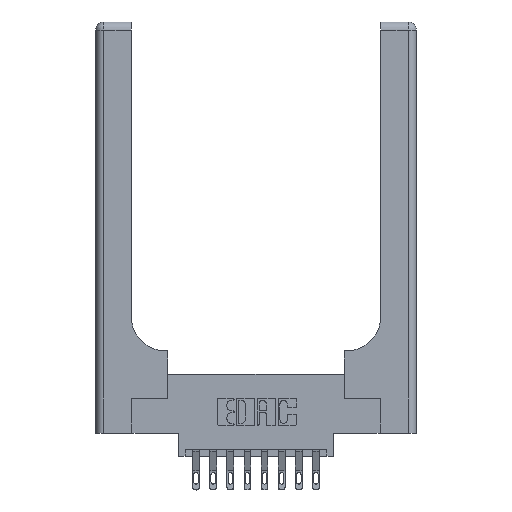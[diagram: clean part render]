
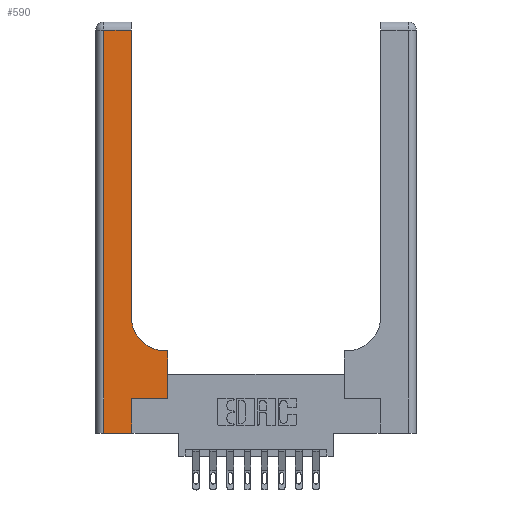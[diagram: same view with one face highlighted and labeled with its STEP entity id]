
A CAD part, top view. The second image highlights one B-rep face of the part: STEP entity #590.
In plain terms, the highlighted planar face has unit normal (0, 0, 1).
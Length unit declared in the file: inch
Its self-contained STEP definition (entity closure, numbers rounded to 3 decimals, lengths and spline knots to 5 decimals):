
#81 = EDGE_CURVE ( 'NONE', #1484, #11618, #7981, .T. ) ;
#280 = CARTESIAN_POINT ( 'NONE',  ( 0., 0., 0.37 ) ) ;
#590 = ADVANCED_FACE ( 'NONE', ( #7961 ), #4794, .F. ) ;
#800 = DIRECTION ( 'NONE',  ( 1., 0., 0. ) ) ;
#896 = DIRECTION ( 'NONE',  ( -1., 0., 0. ) ) ;
#905 = CARTESIAN_POINT ( 'NONE',  ( 0.265, 0.25, 0.37 ) ) ;
#910 = ORIENTED_EDGE ( 'NONE', *, *, #5047, .T. ) ;
#1052 = VERTEX_POINT ( 'NONE', #12951 ) ;
#1266 = DIRECTION ( 'NONE',  ( 0., 0., -1. ) ) ;
#1388 = EDGE_CURVE ( 'NONE', #11535, #1052, #4570, .T. ) ;
#1484 = VERTEX_POINT ( 'NONE', #10128 ) ;
#1550 = DIRECTION ( 'NONE',  ( 0., 1., 0. ) ) ;
#1684 = LINE ( 'NONE', #8360, #4075 ) ;
#1710 = VECTOR ( 'NONE', #4745, 39.37008 ) ;
#1791 = VERTEX_POINT ( 'NONE', #9648 ) ;
#2285 = CARTESIAN_POINT ( 'NONE',  ( 0.265, 0., 0.37 ) ) ;
#2487 = VECTOR ( 'NONE', #8658, 39.37008 ) ;
#2792 = VERTEX_POINT ( 'NONE', #9817 ) ;
#2891 = DIRECTION ( 'NONE',  ( 0., 0., -1. ) ) ;
#3193 = DIRECTION ( 'NONE',  ( -1., 0., 0. ) ) ;
#3281 = CARTESIAN_POINT ( 'NONE',  ( 0.528, 0.25, 0.37 ) ) ;
#3993 = AXIS2_PLACEMENT_3D ( 'NONE', #7188, #1266, #9568 ) ;
#4075 = VECTOR ( 'NONE', #9526, 39.37008 ) ;
#4158 = ORIENTED_EDGE ( 'NONE', *, *, #7753, .T. ) ;
#4262 = ORIENTED_EDGE ( 'NONE', *, *, #1388, .T. ) ;
#4387 = EDGE_LOOP ( 'NONE', ( #6330, #910, #13147, #4158, #7030, #7218, #5301, #10379, #4262 ) ) ;
#4423 = AXIS2_PLACEMENT_3D ( 'NONE', #10025, #2891, #11206 ) ;
#4570 = CIRCLE ( 'NONE', #4423, 0.25 ) ;
#4745 = DIRECTION ( 'NONE',  ( 0., 1., 0. ) ) ;
#4765 = EDGE_CURVE ( 'NONE', #1052, #2792, #15086, .T. ) ;
#4794 = PLANE ( 'NONE',  #3993 ) ;
#4979 = EDGE_CURVE ( 'NONE', #12647, #11535, #6161, .T. ) ;
#5047 = EDGE_CURVE ( 'NONE', #2792, #11682, #5392, .T. ) ;
#5301 = ORIENTED_EDGE ( 'NONE', *, *, #8761, .T. ) ;
#5384 = CARTESIAN_POINT ( 'NONE',  ( 0.528, 0.25, 0.37 ) ) ;
#5392 = LINE ( 'NONE', #15155, #11354 ) ;
#5433 = CARTESIAN_POINT ( 'NONE',  ( 0.06, 0., 0.37 ) ) ;
#5598 = VECTOR ( 'NONE', #1550, 39.37008 ) ;
#6161 = LINE ( 'NONE', #9143, #13585 ) ;
#6330 = ORIENTED_EDGE ( 'NONE', *, *, #4765, .T. ) ;
#6571 = EDGE_CURVE ( 'NONE', #1791, #1484, #7531, .T. ) ;
#6955 = VERTEX_POINT ( 'NONE', #5433 ) ;
#7030 = ORIENTED_EDGE ( 'NONE', *, *, #6571, .T. ) ;
#7188 = CARTESIAN_POINT ( 'NONE',  ( 0., 3., 0.37 ) ) ;
#7218 = ORIENTED_EDGE ( 'NONE', *, *, #81, .T. ) ;
#7468 = CARTESIAN_POINT ( 'NONE',  ( 0.26, 3., 0.37 ) ) ;
#7531 = LINE ( 'NONE', #2285, #14234 ) ;
#7753 = EDGE_CURVE ( 'NONE', #6955, #1791, #8077, .T. ) ;
#7961 = FACE_OUTER_BOUND ( 'NONE', #4387, .T. ) ;
#7981 = LINE ( 'NONE', #905, #13921 ) ;
#8077 = LINE ( 'NONE', #280, #2487 ) ;
#8360 = CARTESIAN_POINT ( 'NONE',  ( 0.06, 3., 0.37 ) ) ;
#8658 = DIRECTION ( 'NONE',  ( 1., 0., 0. ) ) ;
#8761 = EDGE_CURVE ( 'NONE', #11618, #12647, #14361, .T. ) ;
#9143 = CARTESIAN_POINT ( 'NONE',  ( 0.26, 0.6, 0.37 ) ) ;
#9526 = DIRECTION ( 'NONE',  ( 0., -1., 0. ) ) ;
#9568 = DIRECTION ( 'NONE',  ( -1., 0., 0. ) ) ;
#9648 = CARTESIAN_POINT ( 'NONE',  ( 0.265, 0., 0.37 ) ) ;
#9817 = CARTESIAN_POINT ( 'NONE',  ( 0.26, 2.94, 0.37 ) ) ;
#10025 = CARTESIAN_POINT ( 'NONE',  ( 0.51, 0.85, 0.37 ) ) ;
#10128 = CARTESIAN_POINT ( 'NONE',  ( 0.265, 0.25, 0.37 ) ) ;
#10379 = ORIENTED_EDGE ( 'NONE', *, *, #4979, .T. ) ;
#10554 = EDGE_CURVE ( 'NONE', #11682, #6955, #1684, .T. ) ;
#11206 = DIRECTION ( 'NONE',  ( 1., 0., 0. ) ) ;
#11354 = VECTOR ( 'NONE', #896, 39.37008 ) ;
#11479 = CARTESIAN_POINT ( 'NONE',  ( 0.06, 2.94, 0.37 ) ) ;
#11535 = VERTEX_POINT ( 'NONE', #12368 ) ;
#11618 = VERTEX_POINT ( 'NONE', #5384 ) ;
#11682 = VERTEX_POINT ( 'NONE', #11479 ) ;
#11802 = DIRECTION ( 'NONE',  ( 0., 1., 0. ) ) ;
#12368 = CARTESIAN_POINT ( 'NONE',  ( 0.51, 0.6, 0.37 ) ) ;
#12647 = VERTEX_POINT ( 'NONE', #14508 ) ;
#12951 = CARTESIAN_POINT ( 'NONE',  ( 0.26, 0.85, 0.37 ) ) ;
#13147 = ORIENTED_EDGE ( 'NONE', *, *, #10554, .T. ) ;
#13585 = VECTOR ( 'NONE', #3193, 39.37008 ) ;
#13921 = VECTOR ( 'NONE', #800, 39.37008 ) ;
#14234 = VECTOR ( 'NONE', #11802, 39.37008 ) ;
#14361 = LINE ( 'NONE', #3281, #1710 ) ;
#14508 = CARTESIAN_POINT ( 'NONE',  ( 0.528, 0.6, 0.37 ) ) ;
#15086 = LINE ( 'NONE', #7468, #5598 ) ;
#15155 = CARTESIAN_POINT ( 'NONE',  ( 0., 2.94, 0.37 ) ) ;
